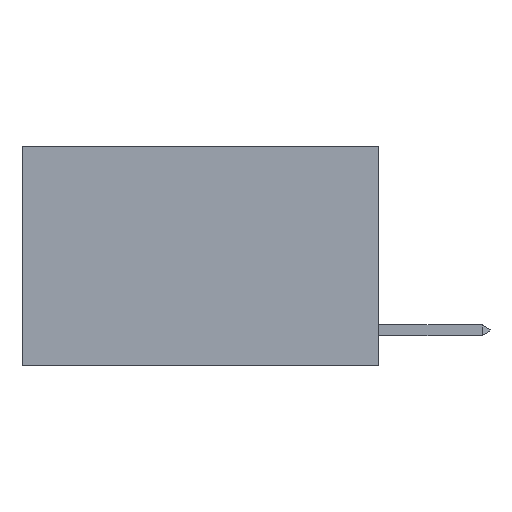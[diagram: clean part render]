
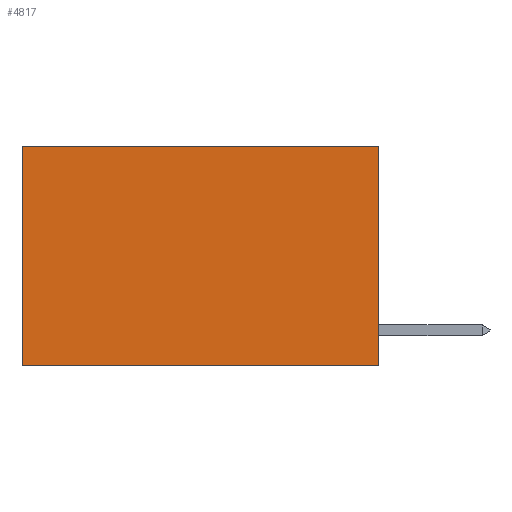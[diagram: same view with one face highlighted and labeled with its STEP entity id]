
A CAD part, left-side view. The second image highlights one B-rep face of the part: STEP entity #4817.
In plain terms, the highlighted planar face has unit normal (-1, 0, 0).
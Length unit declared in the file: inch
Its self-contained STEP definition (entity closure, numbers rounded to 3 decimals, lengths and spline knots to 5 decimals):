
#325 = DIRECTION ( 'NONE',  ( 0., 0., -1. ) ) ;
#560 = EDGE_CURVE ( 'NONE', #13379, #16513, #14330, .T. ) ;
#1020 = VECTOR ( 'NONE', #19262, 39.37008 ) ;
#1443 = LINE ( 'NONE', #11991, #4800 ) ;
#2036 = EDGE_CURVE ( 'NONE', #10787, #13379, #6662, .T. ) ;
#4800 = VECTOR ( 'NONE', #18104, 39.37008 ) ;
#4817 = ADVANCED_FACE ( 'NONE', ( #21876 ), #20347, .F. ) ;
#5373 = CARTESIAN_POINT ( 'NONE',  ( 0.2625, 0., -0.37 ) ) ;
#5468 = EDGE_CURVE ( 'NONE', #21191, #16513, #1443, .T. ) ;
#5632 = ORIENTED_EDGE ( 'NONE', *, *, #2036, .F. ) ;
#5703 = AXIS2_PLACEMENT_3D ( 'NONE', #11289, #14917, #325 ) ;
#6662 = LINE ( 'NONE', #9911, #23134 ) ;
#7943 = ORIENTED_EDGE ( 'NONE', *, *, #560, .F. ) ;
#9809 = LINE ( 'NONE', #22692, #1020 ) ;
#9911 = CARTESIAN_POINT ( 'NONE',  ( 0.2625, 0., 0. ) ) ;
#10787 = VERTEX_POINT ( 'NONE', #12237 ) ;
#11289 = CARTESIAN_POINT ( 'NONE',  ( 0.2625, 0., 0. ) ) ;
#11301 = EDGE_CURVE ( 'NONE', #10787, #21191, #9809, .T. ) ;
#11500 = EDGE_LOOP ( 'NONE', ( #12870, #7943, #5632, #12759 ) ) ;
#11991 = CARTESIAN_POINT ( 'NONE',  ( 0.2625, 0.6, 0. ) ) ;
#12064 = CARTESIAN_POINT ( 'NONE',  ( 0.2625, 0.6, -0.37 ) ) ;
#12237 = CARTESIAN_POINT ( 'NONE',  ( 0.2625, 0., 0. ) ) ;
#12759 = ORIENTED_EDGE ( 'NONE', *, *, #11301, .T. ) ;
#12870 = ORIENTED_EDGE ( 'NONE', *, *, #5468, .T. ) ;
#13379 = VERTEX_POINT ( 'NONE', #5373 ) ;
#14330 = LINE ( 'NONE', #16043, #21401 ) ;
#14917 = DIRECTION ( 'NONE',  ( 1., 0., 0. ) ) ;
#15224 = DIRECTION ( 'NONE',  ( 0., 0., -1. ) ) ;
#16043 = CARTESIAN_POINT ( 'NONE',  ( 0.2625, 0., -0.37 ) ) ;
#16513 = VERTEX_POINT ( 'NONE', #12064 ) ;
#17116 = DIRECTION ( 'NONE',  ( 0., 1., 0. ) ) ;
#18104 = DIRECTION ( 'NONE',  ( 0., 0., -1. ) ) ;
#19262 = DIRECTION ( 'NONE',  ( 0., 1., 0. ) ) ;
#20347 = PLANE ( 'NONE',  #5703 ) ;
#21191 = VERTEX_POINT ( 'NONE', #22058 ) ;
#21401 = VECTOR ( 'NONE', #17116, 39.37008 ) ;
#21876 = FACE_OUTER_BOUND ( 'NONE', #11500, .T. ) ;
#22058 = CARTESIAN_POINT ( 'NONE',  ( 0.2625, 0.6, 0. ) ) ;
#22692 = CARTESIAN_POINT ( 'NONE',  ( 0.2625, 0., 0. ) ) ;
#23134 = VECTOR ( 'NONE', #15224, 39.37008 ) ;
